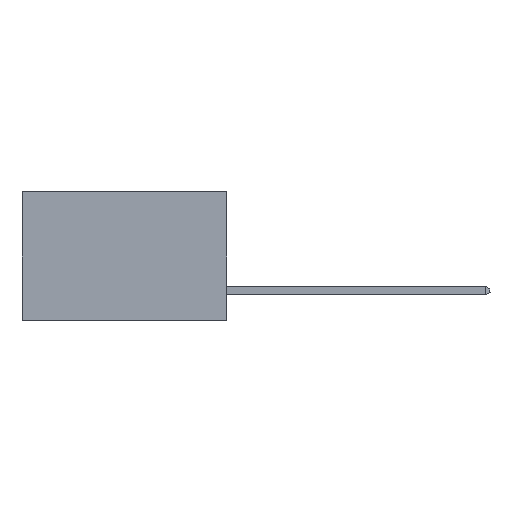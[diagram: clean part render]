
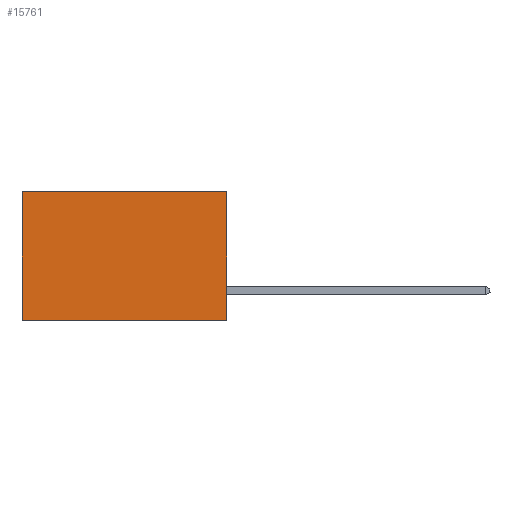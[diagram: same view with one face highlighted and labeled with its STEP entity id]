
A CAD part, left-side view. The second image highlights one B-rep face of the part: STEP entity #15761.
In plain terms, the highlighted planar face has unit normal (-1, 0, 0).
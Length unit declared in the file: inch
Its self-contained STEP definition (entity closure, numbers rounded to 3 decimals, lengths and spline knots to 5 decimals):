
#196 = ORIENTED_EDGE ( 'NONE', *, *, #13982, .F. ) ;
#295 = LINE ( 'NONE', #19018, #18079 ) ;
#2014 = VERTEX_POINT ( 'NONE', #7361 ) ;
#3157 = ORIENTED_EDGE ( 'NONE', *, *, #28309, .T. ) ;
#3295 = DIRECTION ( 'NONE',  ( 0., 0., -1. ) ) ;
#5987 = VECTOR ( 'NONE', #15963, 39.37008 ) ;
#7361 = CARTESIAN_POINT ( 'NONE',  ( 0.277, 0., -0.37 ) ) ;
#7906 = CARTESIAN_POINT ( 'NONE',  ( 0.277, 0.59, 0. ) ) ;
#10770 = VECTOR ( 'NONE', #30337, 39.37008 ) ;
#11068 = EDGE_CURVE ( 'NONE', #19588, #29120, #25125, .T. ) ;
#12370 = CARTESIAN_POINT ( 'NONE',  ( 0.277, 0.59, -0.37 ) ) ;
#13558 = CARTESIAN_POINT ( 'NONE',  ( 0.277, 0.59, -0.37 ) ) ;
#13982 = EDGE_CURVE ( 'NONE', #19260, #2014, #15633, .T. ) ;
#14489 = FACE_OUTER_BOUND ( 'NONE', #21073, .T. ) ;
#14889 = VECTOR ( 'NONE', #21972, 39.37008 ) ;
#15310 = PLANE ( 'NONE',  #21831 ) ;
#15633 = LINE ( 'NONE', #21422, #14889 ) ;
#15761 = ADVANCED_FACE ( 'NONE', ( #14489 ), #15310, .F. ) ;
#15963 = DIRECTION ( 'NONE',  ( 0., 0., -1. ) ) ;
#17688 = DIRECTION ( 'NONE',  ( 1., 0., 0. ) ) ;
#18079 = VECTOR ( 'NONE', #21446, 39.37008 ) ;
#19018 = CARTESIAN_POINT ( 'NONE',  ( 0.277, 0., 0. ) ) ;
#19260 = VERTEX_POINT ( 'NONE', #25905 ) ;
#19588 = VERTEX_POINT ( 'NONE', #7906 ) ;
#20407 = EDGE_CURVE ( 'NONE', #2014, #29120, #28310, .T. ) ;
#21073 = EDGE_LOOP ( 'NONE', ( #25471, #21451, #196, #3157 ) ) ;
#21422 = CARTESIAN_POINT ( 'NONE',  ( 0.277, 0., -0.37 ) ) ;
#21446 = DIRECTION ( 'NONE',  ( 0., 1., 0. ) ) ;
#21451 = ORIENTED_EDGE ( 'NONE', *, *, #20407, .F. ) ;
#21831 = AXIS2_PLACEMENT_3D ( 'NONE', #29517, #17688, #3295 ) ;
#21972 = DIRECTION ( 'NONE',  ( 0., 0., -1. ) ) ;
#25125 = LINE ( 'NONE', #13558, #5987 ) ;
#25471 = ORIENTED_EDGE ( 'NONE', *, *, #11068, .T. ) ;
#25905 = CARTESIAN_POINT ( 'NONE',  ( 0.277, 0., 0. ) ) ;
#27994 = CARTESIAN_POINT ( 'NONE',  ( 0.277, 0., -0.37 ) ) ;
#28309 = EDGE_CURVE ( 'NONE', #19260, #19588, #295, .T. ) ;
#28310 = LINE ( 'NONE', #27994, #10770 ) ;
#29120 = VERTEX_POINT ( 'NONE', #12370 ) ;
#29517 = CARTESIAN_POINT ( 'NONE',  ( 0.277, 0., -0.37 ) ) ;
#30337 = DIRECTION ( 'NONE',  ( 0., 1., 0. ) ) ;
